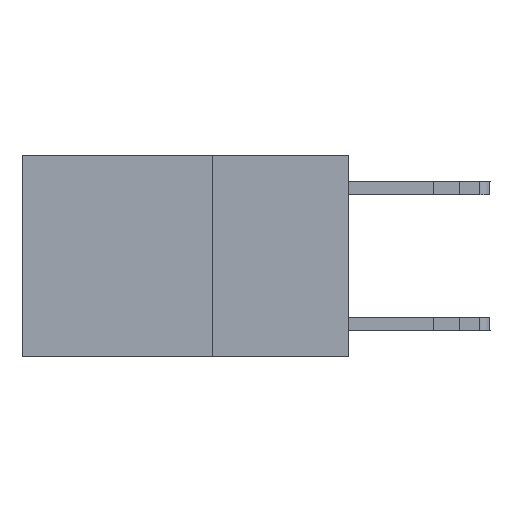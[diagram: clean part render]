
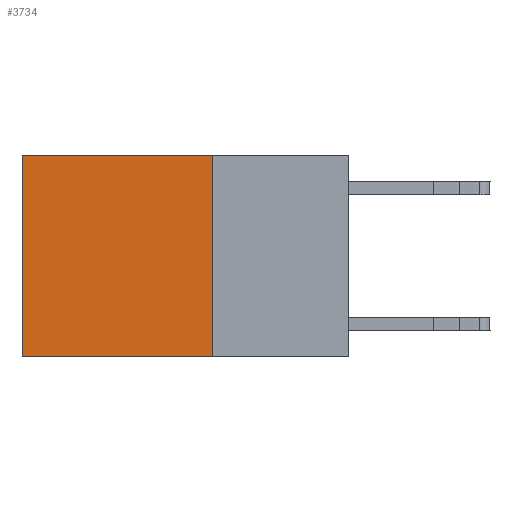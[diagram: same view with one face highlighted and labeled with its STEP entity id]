
A CAD part, left-side view. The second image highlights one B-rep face of the part: STEP entity #3734.
In plain terms, the highlighted planar face has unit normal (-1, 0, 0).
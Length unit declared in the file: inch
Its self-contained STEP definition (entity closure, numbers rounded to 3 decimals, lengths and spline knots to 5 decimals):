
#150 = DIRECTION ( 'NONE',  ( 0., 0., -1. ) ) ;
#2776 = CARTESIAN_POINT ( 'NONE',  ( 0.2625, 0.25, 0. ) ) ;
#2787 = VECTOR ( 'NONE', #150, 39.37008 ) ;
#2846 = LINE ( 'NONE', #6077, #12334 ) ;
#3087 = EDGE_CURVE ( 'NONE', #17770, #13586, #2846, .T. ) ;
#3734 = ADVANCED_FACE ( 'NONE', ( #16076 ), #12618, .F. ) ;
#4447 = VECTOR ( 'NONE', #10040, 39.37008 ) ;
#4660 = EDGE_LOOP ( 'NONE', ( #5298, #9976, #20287, #9354 ) ) ;
#5298 = ORIENTED_EDGE ( 'NONE', *, *, #18405, .T. ) ;
#6077 = CARTESIAN_POINT ( 'NONE',  ( 0.2625, 0.25, 0. ) ) ;
#6890 = CARTESIAN_POINT ( 'NONE',  ( 0.2625, 0.25, -0.37 ) ) ;
#7797 = CARTESIAN_POINT ( 'NONE',  ( 0.2625, 0.6, -0.37 ) ) ;
#7804 = CARTESIAN_POINT ( 'NONE',  ( 0.2625, 0.25, 0. ) ) ;
#8319 = VERTEX_POINT ( 'NONE', #18591 ) ;
#9354 = ORIENTED_EDGE ( 'NONE', *, *, #3087, .T. ) ;
#9976 = ORIENTED_EDGE ( 'NONE', *, *, #10553, .F. ) ;
#10040 = DIRECTION ( 'NONE',  ( 0., 1., 0. ) ) ;
#10553 = EDGE_CURVE ( 'NONE', #8319, #15644, #13603, .T. ) ;
#10730 = DIRECTION ( 'NONE',  ( 1., 0., 0. ) ) ;
#11773 = EDGE_CURVE ( 'NONE', #17770, #8319, #14512, .T. ) ;
#12334 = VECTOR ( 'NONE', #14808, 39.37008 ) ;
#12618 = PLANE ( 'NONE',  #20133 ) ;
#13586 = VERTEX_POINT ( 'NONE', #16003 ) ;
#13603 = LINE ( 'NONE', #6890, #4447 ) ;
#13896 = LINE ( 'NONE', #17258, #2787 ) ;
#14512 = LINE ( 'NONE', #2776, #16318 ) ;
#14808 = DIRECTION ( 'NONE',  ( 0., 1., 0. ) ) ;
#15639 = DIRECTION ( 'NONE',  ( 0., 0., -1. ) ) ;
#15644 = VERTEX_POINT ( 'NONE', #7797 ) ;
#16003 = CARTESIAN_POINT ( 'NONE',  ( 0.2625, 0.6, 0. ) ) ;
#16076 = FACE_OUTER_BOUND ( 'NONE', #4660, .T. ) ;
#16318 = VECTOR ( 'NONE', #21785, 39.37008 ) ;
#17258 = CARTESIAN_POINT ( 'NONE',  ( 0.2625, 0.6, 0. ) ) ;
#17770 = VERTEX_POINT ( 'NONE', #7804 ) ;
#18405 = EDGE_CURVE ( 'NONE', #13586, #15644, #13896, .T. ) ;
#18591 = CARTESIAN_POINT ( 'NONE',  ( 0.2625, 0.25, -0.37 ) ) ;
#19334 = CARTESIAN_POINT ( 'NONE',  ( 0.2625, 0.25, 0. ) ) ;
#20133 = AXIS2_PLACEMENT_3D ( 'NONE', #19334, #10730, #15639 ) ;
#20287 = ORIENTED_EDGE ( 'NONE', *, *, #11773, .F. ) ;
#21785 = DIRECTION ( 'NONE',  ( 0., 0., -1. ) ) ;
